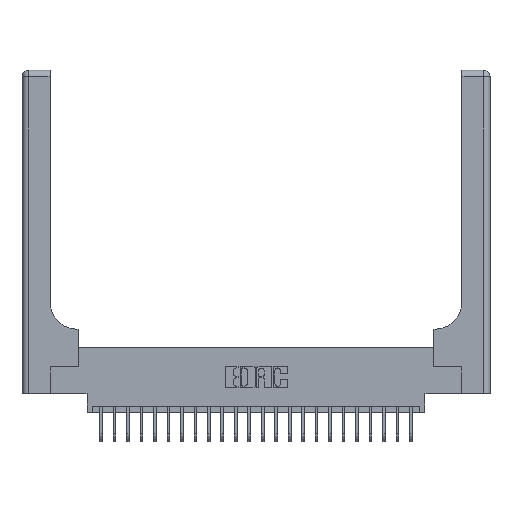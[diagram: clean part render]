
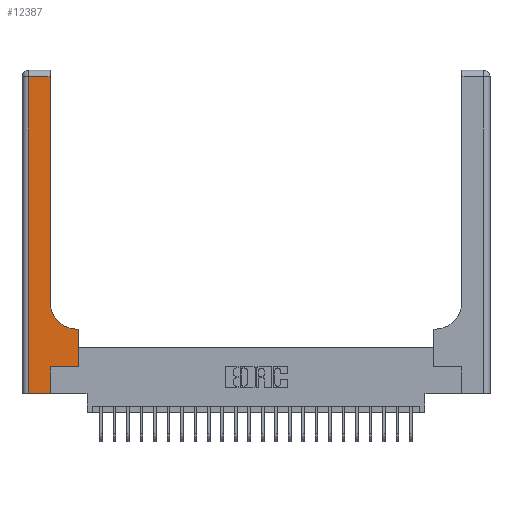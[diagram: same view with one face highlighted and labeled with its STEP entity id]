
A CAD part, top view. The second image highlights one B-rep face of the part: STEP entity #12387.
In plain terms, the highlighted planar face has unit normal (0, 0, 1).
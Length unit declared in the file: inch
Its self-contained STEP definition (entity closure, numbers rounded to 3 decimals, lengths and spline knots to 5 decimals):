
#31 = EDGE_CURVE ( 'NONE', #10182, #4686, #20593, .T. ) ;
#102 = CARTESIAN_POINT ( 'NONE',  ( 0.265, 0., 0.37 ) ) ;
#132 = EDGE_CURVE ( 'NONE', #8111, #22614, #4449, .T. ) ;
#485 = DIRECTION ( 'NONE',  ( -1., 0., 0. ) ) ;
#955 = ORIENTED_EDGE ( 'NONE', *, *, #3454, .T. ) ;
#1188 = CARTESIAN_POINT ( 'NONE',  ( 0.528, 0.25, 0.37 ) ) ;
#1315 = FACE_OUTER_BOUND ( 'NONE', #24506, .T. ) ;
#1551 = DIRECTION ( 'NONE',  ( -1., 0., 0. ) ) ;
#1860 = VECTOR ( 'NONE', #9539, 39.37008 ) ;
#2972 = VERTEX_POINT ( 'NONE', #102 ) ;
#3009 = EDGE_CURVE ( 'NONE', #23497, #11340, #10725, .T. ) ;
#3100 = ORIENTED_EDGE ( 'NONE', *, *, #9631, .T. ) ;
#3281 = CARTESIAN_POINT ( 'NONE',  ( 0., 2.94, 0.37 ) ) ;
#3354 = VECTOR ( 'NONE', #13149, 39.37008 ) ;
#3454 = EDGE_CURVE ( 'NONE', #2972, #23497, #22268, .T. ) ;
#3637 = CARTESIAN_POINT ( 'NONE',  ( 0.528, 0.25, 0.37 ) ) ;
#3773 = DIRECTION ( 'NONE',  ( 1., 0., 0. ) ) ;
#3901 = AXIS2_PLACEMENT_3D ( 'NONE', #14397, #12625, #20384 ) ;
#4449 = LINE ( 'NONE', #3281, #24545 ) ;
#4602 = CARTESIAN_POINT ( 'NONE',  ( 0.51, 0.6, 0.37 ) ) ;
#4627 = DIRECTION ( 'NONE',  ( -1., 0., 0. ) ) ;
#4686 = VERTEX_POINT ( 'NONE', #4602 ) ;
#4887 = VECTOR ( 'NONE', #5766, 39.37008 ) ;
#5766 = DIRECTION ( 'NONE',  ( 1., 0., 0. ) ) ;
#6335 = ORIENTED_EDGE ( 'NONE', *, *, #31, .T. ) ;
#6452 = VECTOR ( 'NONE', #3773, 39.37008 ) ;
#6680 = CARTESIAN_POINT ( 'NONE',  ( 0.26, 0.6, 0.37 ) ) ;
#7512 = VECTOR ( 'NONE', #4627, 39.37008 ) ;
#8034 = EDGE_CURVE ( 'NONE', #4686, #24585, #20156, .T. ) ;
#8111 = VERTEX_POINT ( 'NONE', #12448 ) ;
#9219 = ORIENTED_EDGE ( 'NONE', *, *, #13791, .T. ) ;
#9518 = CARTESIAN_POINT ( 'NONE',  ( 0.265, 0., 0.37 ) ) ;
#9539 = DIRECTION ( 'NONE',  ( 0., 1., 0. ) ) ;
#9631 = EDGE_CURVE ( 'NONE', #22614, #24283, #11558, .T. ) ;
#10182 = VERTEX_POINT ( 'NONE', #10560 ) ;
#10560 = CARTESIAN_POINT ( 'NONE',  ( 0.528, 0.6, 0.37 ) ) ;
#10605 = ORIENTED_EDGE ( 'NONE', *, *, #20420, .T. ) ;
#10725 = LINE ( 'NONE', #19297, #6452 ) ;
#11340 = VERTEX_POINT ( 'NONE', #1188 ) ;
#11558 = LINE ( 'NONE', #12603, #24633 ) ;
#11794 = CARTESIAN_POINT ( 'NONE',  ( 0.26, 3., 0.37 ) ) ;
#12078 = ORIENTED_EDGE ( 'NONE', *, *, #8034, .T. ) ;
#12127 = CARTESIAN_POINT ( 'NONE',  ( 0.265, 0.25, 0.37 ) ) ;
#12387 = ADVANCED_FACE ( 'NONE', ( #1315 ), #13851, .F. ) ;
#12448 = CARTESIAN_POINT ( 'NONE',  ( 0.26, 2.94, 0.37 ) ) ;
#12603 = CARTESIAN_POINT ( 'NONE',  ( 0.06, 3., 0.37 ) ) ;
#12625 = DIRECTION ( 'NONE',  ( 0., 0., -1. ) ) ;
#12821 = VECTOR ( 'NONE', #15266, 39.37008 ) ;
#13147 = CARTESIAN_POINT ( 'NONE',  ( 0.06, 2.94, 0.37 ) ) ;
#13149 = DIRECTION ( 'NONE',  ( 0., 1., 0. ) ) ;
#13791 = EDGE_CURVE ( 'NONE', #24585, #8111, #24402, .T. ) ;
#13851 = PLANE ( 'NONE',  #20601 ) ;
#14084 = ORIENTED_EDGE ( 'NONE', *, *, #20103, .T. ) ;
#14397 = CARTESIAN_POINT ( 'NONE',  ( 0.51, 0.85, 0.37 ) ) ;
#15235 = LINE ( 'NONE', #23217, #4887 ) ;
#15266 = DIRECTION ( 'NONE',  ( 0., 1., 0. ) ) ;
#15608 = CARTESIAN_POINT ( 'NONE',  ( 0.06, 0., 0.37 ) ) ;
#15964 = CARTESIAN_POINT ( 'NONE',  ( 0., 3., 0.37 ) ) ;
#16437 = LINE ( 'NONE', #3637, #3354 ) ;
#18607 = DIRECTION ( 'NONE',  ( 0., -1., 0. ) ) ;
#19297 = CARTESIAN_POINT ( 'NONE',  ( 0.265, 0.25, 0.37 ) ) ;
#20103 = EDGE_CURVE ( 'NONE', #24283, #2972, #15235, .T. ) ;
#20155 = ORIENTED_EDGE ( 'NONE', *, *, #3009, .T. ) ;
#20156 = CIRCLE ( 'NONE', #3901, 0.25 ) ;
#20384 = DIRECTION ( 'NONE',  ( 1., 0., 0. ) ) ;
#20420 = EDGE_CURVE ( 'NONE', #11340, #10182, #16437, .T. ) ;
#20593 = LINE ( 'NONE', #6680, #7512 ) ;
#20601 = AXIS2_PLACEMENT_3D ( 'NONE', #15964, #23886, #485 ) ;
#22268 = LINE ( 'NONE', #9518, #12821 ) ;
#22614 = VERTEX_POINT ( 'NONE', #13147 ) ;
#23008 = CARTESIAN_POINT ( 'NONE',  ( 0.26, 0.85, 0.37 ) ) ;
#23217 = CARTESIAN_POINT ( 'NONE',  ( 0., 0., 0.37 ) ) ;
#23497 = VERTEX_POINT ( 'NONE', #12127 ) ;
#23886 = DIRECTION ( 'NONE',  ( 0., 0., -1. ) ) ;
#24283 = VERTEX_POINT ( 'NONE', #15608 ) ;
#24295 = ORIENTED_EDGE ( 'NONE', *, *, #132, .T. ) ;
#24402 = LINE ( 'NONE', #11794, #1860 ) ;
#24506 = EDGE_LOOP ( 'NONE', ( #9219, #24295, #3100, #14084, #955, #20155, #10605, #6335, #12078 ) ) ;
#24545 = VECTOR ( 'NONE', #1551, 39.37008 ) ;
#24585 = VERTEX_POINT ( 'NONE', #23008 ) ;
#24633 = VECTOR ( 'NONE', #18607, 39.37008 ) ;
